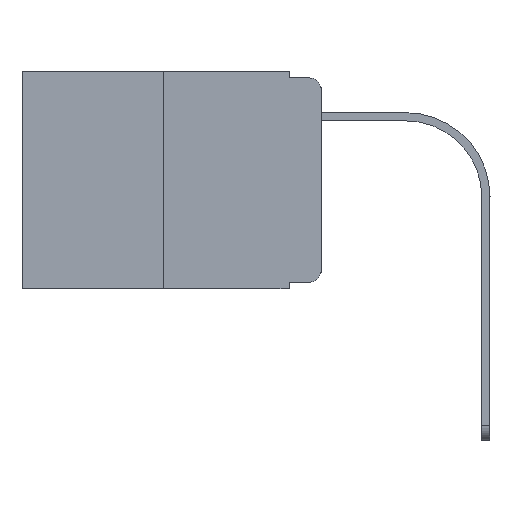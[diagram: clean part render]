
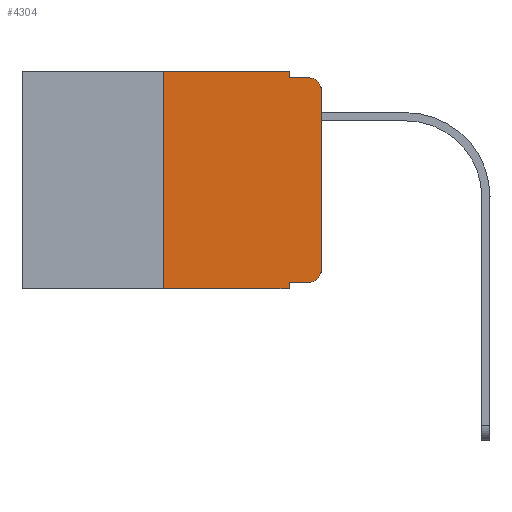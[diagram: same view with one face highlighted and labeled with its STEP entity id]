
A CAD part, left-side view. The second image highlights one B-rep face of the part: STEP entity #4304.
In plain terms, the highlighted planar face has unit normal (-1, 0, 0).
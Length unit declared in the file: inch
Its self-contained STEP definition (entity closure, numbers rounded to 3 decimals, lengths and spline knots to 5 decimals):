
#16 = LINE ( 'NONE', #2364, #9451 ) ;
#104 = CARTESIAN_POINT ( 'NONE',  ( 0., 0.051, 0. ) ) ;
#118 = LINE ( 'NONE', #3332, #8986 ) ;
#198 = ORIENTED_EDGE ( 'NONE', *, *, #8456, .F. ) ;
#231 = EDGE_CURVE ( 'NONE', #3219, #4615, #6544, .T. ) ;
#342 = VERTEX_POINT ( 'NONE', #7293 ) ;
#499 = VERTEX_POINT ( 'NONE', #5272 ) ;
#835 = VECTOR ( 'NONE', #9731, 39.37008 ) ;
#960 = CARTESIAN_POINT ( 'NONE',  ( 0., 0.051, -0.333 ) ) ;
#1200 = PLANE ( 'NONE',  #1938 ) ;
#1212 = CARTESIAN_POINT ( 'NONE',  ( 0., 0.051, 0. ) ) ;
#1224 = CARTESIAN_POINT ( 'NONE',  ( 0., 0.051, -0.01 ) ) ;
#1251 = DIRECTION ( 'NONE',  ( 0., 0., -1. ) ) ;
#1271 = CIRCLE ( 'NONE', #9885, 0.02 ) ;
#1395 = CARTESIAN_POINT ( 'NONE',  ( 0., 0.051, -0.333 ) ) ;
#1914 = CARTESIAN_POINT ( 'NONE',  ( 0., 0.25, 0. ) ) ;
#1927 = FACE_OUTER_BOUND ( 'NONE', #9184, .T. ) ;
#1938 = AXIS2_PLACEMENT_3D ( 'NONE', #3577, #2892, #1251 ) ;
#2364 = CARTESIAN_POINT ( 'NONE',  ( 0., 0.051, -0.01 ) ) ;
#2489 = EDGE_CURVE ( 'NONE', #4414, #342, #7467, .T. ) ;
#2517 = VECTOR ( 'NONE', #9096, 39.37008 ) ;
#2549 = EDGE_CURVE ( 'NONE', #4414, #9772, #118, .T. ) ;
#2712 = ORIENTED_EDGE ( 'NONE', *, *, #231, .F. ) ;
#2892 = DIRECTION ( 'NONE',  ( 1., 0., 0. ) ) ;
#2984 = EDGE_CURVE ( 'NONE', #8161, #6538, #4095, .T. ) ;
#3162 = DIRECTION ( 'NONE',  ( 0., -1., 0. ) ) ;
#3219 = VERTEX_POINT ( 'NONE', #3917 ) ;
#3332 = CARTESIAN_POINT ( 'NONE',  ( 0., 0.051, 0. ) ) ;
#3366 = LINE ( 'NONE', #9768, #3669 ) ;
#3383 = CARTESIAN_POINT ( 'NONE',  ( 0., 0.473, 0. ) ) ;
#3466 = CARTESIAN_POINT ( 'NONE',  ( 0., 0.25, 0. ) ) ;
#3577 = CARTESIAN_POINT ( 'NONE',  ( 0., 0.473, 0. ) ) ;
#3669 = VECTOR ( 'NONE', #6596, 39.37008 ) ;
#3671 = ORIENTED_EDGE ( 'NONE', *, *, #7125, .T. ) ;
#3868 = VERTEX_POINT ( 'NONE', #8624 ) ;
#3917 = CARTESIAN_POINT ( 'NONE',  ( 0., 0.25, -0.343 ) ) ;
#4025 = AXIS2_PLACEMENT_3D ( 'NONE', #9473, #4545, #9377 ) ;
#4068 = DIRECTION ( 'NONE',  ( 0., 0., -1. ) ) ;
#4095 = LINE ( 'NONE', #104, #10061 ) ;
#4127 = ORIENTED_EDGE ( 'NONE', *, *, #8469, .F. ) ;
#4213 = VECTOR ( 'NONE', #9932, 39.37008 ) ;
#4304 = ADVANCED_FACE ( 'NONE', ( #1927 ), #1200, .F. ) ;
#4414 = VERTEX_POINT ( 'NONE', #1395 ) ;
#4457 = VERTEX_POINT ( 'NONE', #9455 ) ;
#4464 = ORIENTED_EDGE ( 'NONE', *, *, #2549, .F. ) ;
#4545 = DIRECTION ( 'NONE',  ( -1., 0., 0. ) ) ;
#4615 = VERTEX_POINT ( 'NONE', #3466 ) ;
#5115 = DIRECTION ( 'NONE',  ( 0., 0., 1. ) ) ;
#5272 = CARTESIAN_POINT ( 'NONE',  ( 0., 0.02, -0.01 ) ) ;
#6001 = EDGE_CURVE ( 'NONE', #3219, #9772, #3366, .T. ) ;
#6400 = CARTESIAN_POINT ( 'NONE',  ( 0., 0.051, -0.343 ) ) ;
#6411 = CARTESIAN_POINT ( 'NONE',  ( 0., 0.02, -0.313 ) ) ;
#6538 = VERTEX_POINT ( 'NONE', #1224 ) ;
#6544 = LINE ( 'NONE', #1914, #9369 ) ;
#6559 = DIRECTION ( 'NONE',  ( 0., 0., -1. ) ) ;
#6596 = DIRECTION ( 'NONE',  ( 0., -1., 0. ) ) ;
#6620 = DIRECTION ( 'NONE',  ( -1., 0., 0. ) ) ;
#6646 = LINE ( 'NONE', #10355, #2517 ) ;
#7125 = EDGE_CURVE ( 'NONE', #3868, #499, #8788, .T. ) ;
#7230 = EDGE_CURVE ( 'NONE', #4457, #3868, #6646, .T. ) ;
#7293 = CARTESIAN_POINT ( 'NONE',  ( 0., 0.02, -0.333 ) ) ;
#7467 = LINE ( 'NONE', #960, #4213 ) ;
#8161 = VERTEX_POINT ( 'NONE', #1212 ) ;
#8243 = ORIENTED_EDGE ( 'NONE', *, *, #7230, .T. ) ;
#8456 = EDGE_CURVE ( 'NONE', #6538, #499, #16, .T. ) ;
#8469 = EDGE_CURVE ( 'NONE', #4615, #8161, #8962, .T. ) ;
#8493 = ORIENTED_EDGE ( 'NONE', *, *, #9234, .T. ) ;
#8624 = CARTESIAN_POINT ( 'NONE',  ( 0., 0., -0.03 ) ) ;
#8788 = CIRCLE ( 'NONE', #4025, 0.02 ) ;
#8833 = ORIENTED_EDGE ( 'NONE', *, *, #2489, .T. ) ;
#8962 = LINE ( 'NONE', #3383, #835 ) ;
#8986 = VECTOR ( 'NONE', #6559, 39.37008 ) ;
#9096 = DIRECTION ( 'NONE',  ( 0., 0., 1. ) ) ;
#9184 = EDGE_LOOP ( 'NONE', ( #8243, #3671, #198, #9563, #4127, #2712, #10192, #4464, #8833, #8493 ) ) ;
#9234 = EDGE_CURVE ( 'NONE', #342, #4457, #1271, .T. ) ;
#9369 = VECTOR ( 'NONE', #5115, 39.37008 ) ;
#9377 = DIRECTION ( 'NONE',  ( 0., 0., -1. ) ) ;
#9451 = VECTOR ( 'NONE', #3162, 39.37008 ) ;
#9455 = CARTESIAN_POINT ( 'NONE',  ( 0., 0., -0.313 ) ) ;
#9473 = CARTESIAN_POINT ( 'NONE',  ( 0., 0.02, -0.03 ) ) ;
#9563 = ORIENTED_EDGE ( 'NONE', *, *, #2984, .F. ) ;
#9731 = DIRECTION ( 'NONE',  ( 0., -1., 0. ) ) ;
#9768 = CARTESIAN_POINT ( 'NONE',  ( 0., 0.473, -0.343 ) ) ;
#9772 = VERTEX_POINT ( 'NONE', #6400 ) ;
#9775 = DIRECTION ( 'NONE',  ( 0., 0., -1. ) ) ;
#9885 = AXIS2_PLACEMENT_3D ( 'NONE', #6411, #6620, #4068 ) ;
#9932 = DIRECTION ( 'NONE',  ( 0., -1., 0. ) ) ;
#10061 = VECTOR ( 'NONE', #9775, 39.37008 ) ;
#10192 = ORIENTED_EDGE ( 'NONE', *, *, #6001, .T. ) ;
#10355 = CARTESIAN_POINT ( 'NONE',  ( 0., 0., 0. ) ) ;
